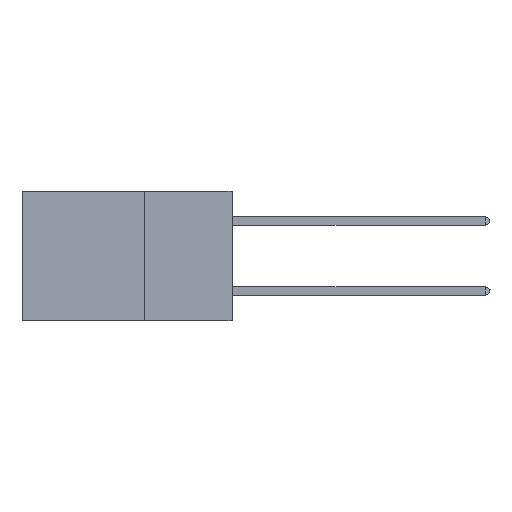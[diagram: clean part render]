
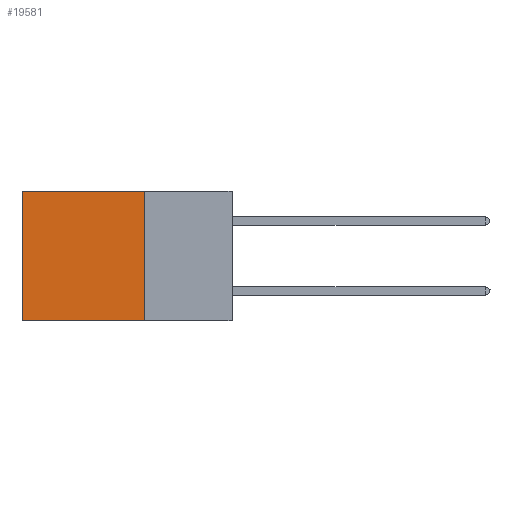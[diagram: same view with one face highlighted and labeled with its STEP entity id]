
A CAD part, left-side view. The second image highlights one B-rep face of the part: STEP entity #19581.
In plain terms, the highlighted planar face has unit normal (-1, 0, 0).
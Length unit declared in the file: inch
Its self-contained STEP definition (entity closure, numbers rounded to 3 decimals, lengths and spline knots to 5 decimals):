
#20 = CARTESIAN_POINT ( 'NONE',  ( 0.2875, 0.25, 0. ) ) ;
#1380 = EDGE_CURVE ( 'NONE', #20236, #15777, #11498, .T. ) ;
#1400 = CARTESIAN_POINT ( 'NONE',  ( 0.2875, 0.6, -0.37 ) ) ;
#2672 = PLANE ( 'NONE',  #32197 ) ;
#4019 = EDGE_CURVE ( 'NONE', #20236, #8117, #35319, .T. ) ;
#4552 = CARTESIAN_POINT ( 'NONE',  ( 0.2875, 0.25, 0. ) ) ;
#4827 = ORIENTED_EDGE ( 'NONE', *, *, #5547, .T. ) ;
#5547 = EDGE_CURVE ( 'NONE', #8117, #18278, #18693, .T. ) ;
#8117 = VERTEX_POINT ( 'NONE', #30528 ) ;
#9247 = DIRECTION ( 'NONE',  ( 0., 0., -1. ) ) ;
#10418 = FACE_OUTER_BOUND ( 'NONE', #26838, .T. ) ;
#10588 = CARTESIAN_POINT ( 'NONE',  ( 0.2875, 0.25, -0.37 ) ) ;
#10810 = DIRECTION ( 'NONE',  ( 0., 0., -1. ) ) ;
#11243 = VECTOR ( 'NONE', #13394, 39.37008 ) ;
#11315 = DIRECTION ( 'NONE',  ( 0., 1., 0. ) ) ;
#11498 = LINE ( 'NONE', #20404, #14991 ) ;
#13394 = DIRECTION ( 'NONE',  ( 0., 1., 0. ) ) ;
#13847 = ORIENTED_EDGE ( 'NONE', *, *, #14588, .F. ) ;
#14588 = EDGE_CURVE ( 'NONE', #15777, #18278, #16064, .T. ) ;
#14991 = VECTOR ( 'NONE', #9247, 39.37008 ) ;
#15777 = VERTEX_POINT ( 'NONE', #27644 ) ;
#16064 = LINE ( 'NONE', #10588, #11243 ) ;
#16184 = CARTESIAN_POINT ( 'NONE',  ( 0.2875, 0.25, 0. ) ) ;
#17042 = CARTESIAN_POINT ( 'NONE',  ( 0.2875, 0.6, 0. ) ) ;
#18278 = VERTEX_POINT ( 'NONE', #1400 ) ;
#18693 = LINE ( 'NONE', #17042, #20860 ) ;
#19083 = ORIENTED_EDGE ( 'NONE', *, *, #1380, .F. ) ;
#19581 = ADVANCED_FACE ( 'NONE', ( #10418 ), #2672, .F. ) ;
#20236 = VERTEX_POINT ( 'NONE', #4552 ) ;
#20404 = CARTESIAN_POINT ( 'NONE',  ( 0.2875, 0.25, 0. ) ) ;
#20860 = VECTOR ( 'NONE', #30419, 39.37008 ) ;
#26838 = EDGE_LOOP ( 'NONE', ( #4827, #13847, #19083, #35190 ) ) ;
#27644 = CARTESIAN_POINT ( 'NONE',  ( 0.2875, 0.25, -0.37 ) ) ;
#27907 = VECTOR ( 'NONE', #11315, 39.37008 ) ;
#30419 = DIRECTION ( 'NONE',  ( 0., 0., -1. ) ) ;
#30528 = CARTESIAN_POINT ( 'NONE',  ( 0.2875, 0.6, 0. ) ) ;
#32197 = AXIS2_PLACEMENT_3D ( 'NONE', #16184, #33095, #10810 ) ;
#33095 = DIRECTION ( 'NONE',  ( 1., 0., 0. ) ) ;
#35190 = ORIENTED_EDGE ( 'NONE', *, *, #4019, .T. ) ;
#35319 = LINE ( 'NONE', #20, #27907 ) ;
